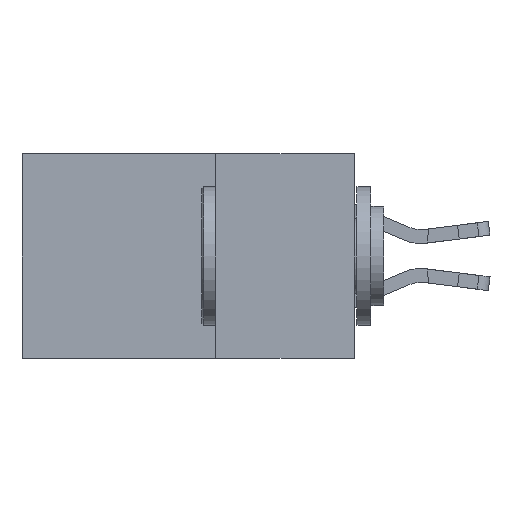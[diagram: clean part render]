
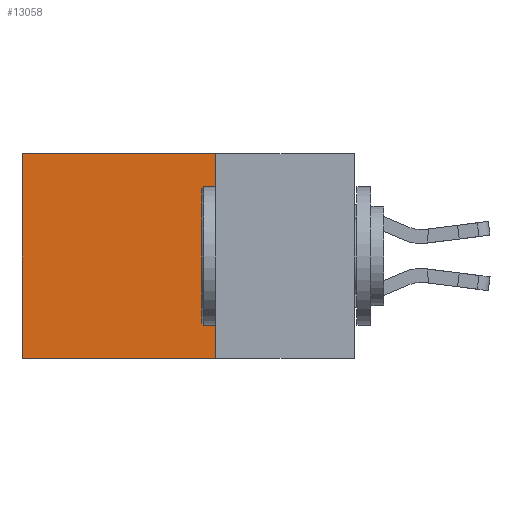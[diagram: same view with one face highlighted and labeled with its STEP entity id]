
A CAD part, left-side view. The second image highlights one B-rep face of the part: STEP entity #13058.
In plain terms, the highlighted planar face has unit normal (-1, 0, 0).
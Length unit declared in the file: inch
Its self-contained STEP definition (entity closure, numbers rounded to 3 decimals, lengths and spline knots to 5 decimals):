
#653 = CARTESIAN_POINT ( 'NONE',  ( 0.2615, 0.6, 0. ) ) ;
#1781 = VERTEX_POINT ( 'NONE', #4497 ) ;
#2151 = ORIENTED_EDGE ( 'NONE', *, *, #9544, .F. ) ;
#3155 = CARTESIAN_POINT ( 'NONE',  ( 0.2615, 0.25, -0.37 ) ) ;
#3285 = VECTOR ( 'NONE', #5093, 39.37008 ) ;
#4497 = CARTESIAN_POINT ( 'NONE',  ( 0.2615, 0.25, 0. ) ) ;
#4822 = EDGE_CURVE ( 'NONE', #1781, #8540, #9884, .T. ) ;
#4916 = LINE ( 'NONE', #9391, #7884 ) ;
#5004 = VERTEX_POINT ( 'NONE', #3155 ) ;
#5093 = DIRECTION ( 'NONE',  ( 0., 1., 0. ) ) ;
#5117 = CARTESIAN_POINT ( 'NONE',  ( 0.2615, 0.25, 0. ) ) ;
#5627 = VECTOR ( 'NONE', #8844, 39.37008 ) ;
#5998 = FACE_OUTER_BOUND ( 'NONE', #7816, .T. ) ;
#6126 = ORIENTED_EDGE ( 'NONE', *, *, #4822, .T. ) ;
#6724 = CARTESIAN_POINT ( 'NONE',  ( 0.2615, 0.6, -0.37 ) ) ;
#7360 = EDGE_CURVE ( 'NONE', #5004, #12069, #9302, .T. ) ;
#7365 = ORIENTED_EDGE ( 'NONE', *, *, #12824, .T. ) ;
#7816 = EDGE_LOOP ( 'NONE', ( #7365, #13468, #2151, #6126 ) ) ;
#7884 = VECTOR ( 'NONE', #9069, 39.37008 ) ;
#8540 = VERTEX_POINT ( 'NONE', #653 ) ;
#8833 = VECTOR ( 'NONE', #13425, 39.37008 ) ;
#8844 = DIRECTION ( 'NONE',  ( 0., 1., 0. ) ) ;
#8901 = CARTESIAN_POINT ( 'NONE',  ( 0.2615, 0.25, -0.37 ) ) ;
#9069 = DIRECTION ( 'NONE',  ( 0., 0., -1. ) ) ;
#9302 = LINE ( 'NONE', #8901, #5627 ) ;
#9391 = CARTESIAN_POINT ( 'NONE',  ( 0.2615, 0.25, -0.37 ) ) ;
#9544 = EDGE_CURVE ( 'NONE', #1781, #5004, #4916, .T. ) ;
#9884 = LINE ( 'NONE', #5117, #3285 ) ;
#11063 = DIRECTION ( 'NONE',  ( 0., 0., -1. ) ) ;
#11076 = DIRECTION ( 'NONE',  ( 1., 0., 0. ) ) ;
#11172 = PLANE ( 'NONE',  #13274 ) ;
#11232 = CARTESIAN_POINT ( 'NONE',  ( 0.2615, 0.25, -0.37 ) ) ;
#11693 = LINE ( 'NONE', #13753, #8833 ) ;
#12069 = VERTEX_POINT ( 'NONE', #6724 ) ;
#12824 = EDGE_CURVE ( 'NONE', #8540, #12069, #11693, .T. ) ;
#13058 = ADVANCED_FACE ( 'NONE', ( #5998 ), #11172, .F. ) ;
#13274 = AXIS2_PLACEMENT_3D ( 'NONE', #11232, #11076, #11063 ) ;
#13425 = DIRECTION ( 'NONE',  ( 0., 0., -1. ) ) ;
#13468 = ORIENTED_EDGE ( 'NONE', *, *, #7360, .F. ) ;
#13753 = CARTESIAN_POINT ( 'NONE',  ( 0.2615, 0.6, -0.37 ) ) ;
